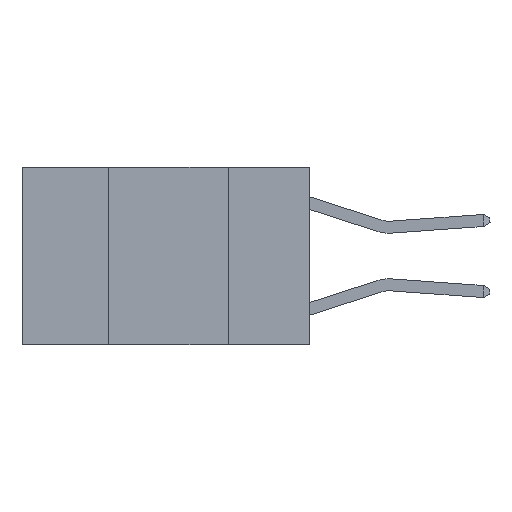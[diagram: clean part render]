
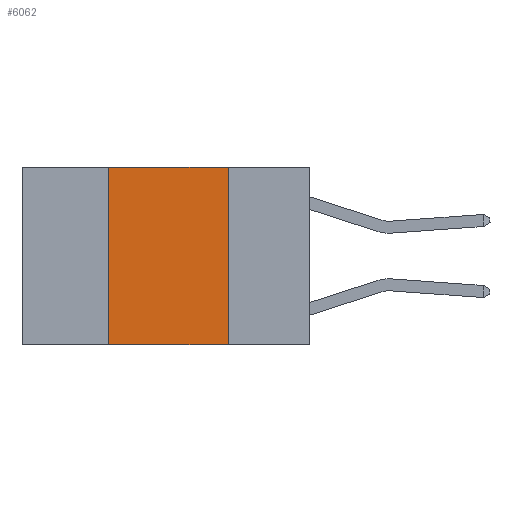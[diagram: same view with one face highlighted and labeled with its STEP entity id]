
A CAD part, left-side view. The second image highlights one B-rep face of the part: STEP entity #6062.
In plain terms, the highlighted planar face has unit normal (-1, 0, 0).
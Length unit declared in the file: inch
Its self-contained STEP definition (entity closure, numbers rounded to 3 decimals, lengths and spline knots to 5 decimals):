
#1325 = EDGE_CURVE ( 'NONE', #7698, #10856, #11119, .T. ) ;
#1567 = EDGE_CURVE ( 'NONE', #11360, #9457, #9616, .T. ) ;
#1714 = VECTOR ( 'NONE', #8292, 39.37008 ) ;
#1744 = EDGE_CURVE ( 'NONE', #11360, #10856, #6132, .T. ) ;
#1916 = LINE ( 'NONE', #2833, #6594 ) ;
#2328 = FACE_OUTER_BOUND ( 'NONE', #3409, .T. ) ;
#2833 = CARTESIAN_POINT ( 'NONE',  ( 0., 0.6, 0. ) ) ;
#2879 = DIRECTION ( 'NONE',  ( 0., -1., 0. ) ) ;
#3386 = CARTESIAN_POINT ( 'NONE',  ( 0., 0.42, 0. ) ) ;
#3409 = EDGE_LOOP ( 'NONE', ( #9078, #9037, #7328, #6294 ) ) ;
#3470 = EDGE_CURVE ( 'NONE', #9457, #7698, #1916, .T. ) ;
#3785 = DIRECTION ( 'NONE',  ( 0., -1., 0. ) ) ;
#5058 = DIRECTION ( 'NONE',  ( 0., 0., -1. ) ) ;
#5368 = CARTESIAN_POINT ( 'NONE',  ( 0., 0.17, 0. ) ) ;
#6062 = ADVANCED_FACE ( 'NONE', ( #2328 ), #8607, .F. ) ;
#6132 = LINE ( 'NONE', #6561, #8180 ) ;
#6294 = ORIENTED_EDGE ( 'NONE', *, *, #1744, .T. ) ;
#6561 = CARTESIAN_POINT ( 'NONE',  ( 0., 0.6, -0.37 ) ) ;
#6594 = VECTOR ( 'NONE', #3785, 39.37008 ) ;
#7328 = ORIENTED_EDGE ( 'NONE', *, *, #1567, .F. ) ;
#7698 = VERTEX_POINT ( 'NONE', #5368 ) ;
#7911 = CARTESIAN_POINT ( 'NONE',  ( 0., 0.42, -0.37 ) ) ;
#8180 = VECTOR ( 'NONE', #2879, 39.37008 ) ;
#8292 = DIRECTION ( 'NONE',  ( 0., 0., -1. ) ) ;
#8607 = PLANE ( 'NONE',  #10465 ) ;
#8744 = DIRECTION ( 'NONE',  ( 0., 0., 1. ) ) ;
#9037 = ORIENTED_EDGE ( 'NONE', *, *, #3470, .F. ) ;
#9078 = ORIENTED_EDGE ( 'NONE', *, *, #1325, .F. ) ;
#9097 = CARTESIAN_POINT ( 'NONE',  ( 0., 0.17, 0. ) ) ;
#9205 = CARTESIAN_POINT ( 'NONE',  ( 0., 0.42, 0. ) ) ;
#9433 = CARTESIAN_POINT ( 'NONE',  ( 0., 0.6, 0. ) ) ;
#9457 = VERTEX_POINT ( 'NONE', #9205 ) ;
#9616 = LINE ( 'NONE', #3386, #11494 ) ;
#9947 = CARTESIAN_POINT ( 'NONE',  ( 0., 0.17, -0.37 ) ) ;
#10238 = DIRECTION ( 'NONE',  ( 1., 0., 0. ) ) ;
#10465 = AXIS2_PLACEMENT_3D ( 'NONE', #9433, #10238, #5058 ) ;
#10856 = VERTEX_POINT ( 'NONE', #9947 ) ;
#11119 = LINE ( 'NONE', #9097, #1714 ) ;
#11360 = VERTEX_POINT ( 'NONE', #7911 ) ;
#11494 = VECTOR ( 'NONE', #8744, 39.37008 ) ;
